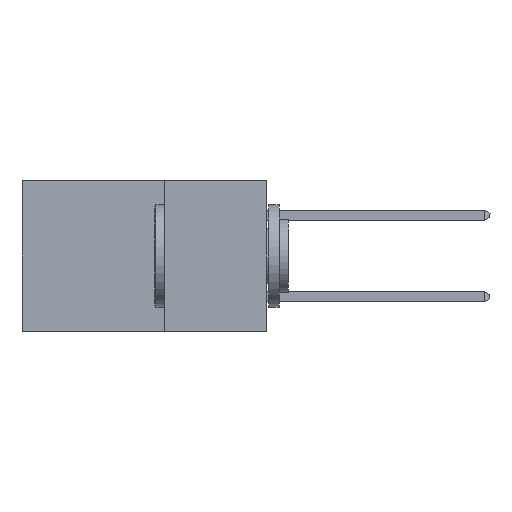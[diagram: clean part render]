
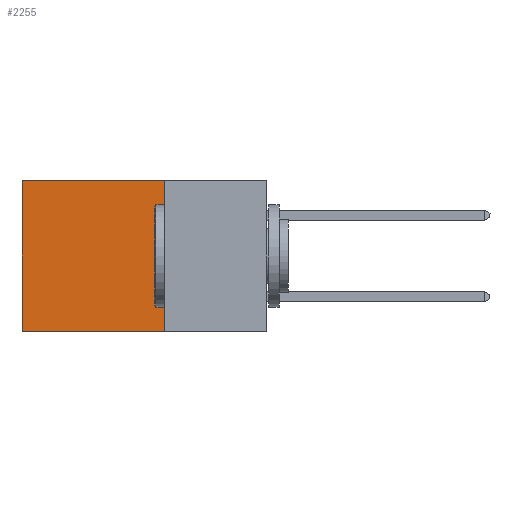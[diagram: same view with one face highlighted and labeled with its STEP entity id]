
A CAD part, left-side view. The second image highlights one B-rep face of the part: STEP entity #2255.
In plain terms, the highlighted planar face has unit normal (-1, 0, 0).
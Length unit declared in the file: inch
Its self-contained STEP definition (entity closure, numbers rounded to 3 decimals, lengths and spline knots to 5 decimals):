
#316 = ORIENTED_EDGE ( 'NONE', *, *, #842, .T. ) ;
#406 = ORIENTED_EDGE ( 'NONE', *, *, #447, .F. ) ;
#423 = VECTOR ( 'NONE', #3662, 39.37008 ) ;
#447 = EDGE_CURVE ( 'NONE', #13994, #11689, #9761, .T. ) ;
#842 = EDGE_CURVE ( 'NONE', #3643, #11689, #13618, .T. ) ;
#846 = VECTOR ( 'NONE', #10991, 39.37008 ) ;
#1042 = LINE ( 'NONE', #2290, #7118 ) ;
#1079 = CARTESIAN_POINT ( 'NONE',  ( 0.2875, 0.6, -0.37 ) ) ;
#1954 = VERTEX_POINT ( 'NONE', #15125 ) ;
#2255 = ADVANCED_FACE ( 'NONE', ( #5760 ), #12206, .F. ) ;
#2290 = CARTESIAN_POINT ( 'NONE',  ( 0.2875, 0.25, 0. ) ) ;
#2698 = AXIS2_PLACEMENT_3D ( 'NONE', #12236, #12100, #12096 ) ;
#3304 = ORIENTED_EDGE ( 'NONE', *, *, #9925, .T. ) ;
#3643 = VERTEX_POINT ( 'NONE', #15155 ) ;
#3662 = DIRECTION ( 'NONE',  ( 0., 1., 0. ) ) ;
#3919 = CARTESIAN_POINT ( 'NONE',  ( 0.2875, 0.25, -0.37 ) ) ;
#4709 = CARTESIAN_POINT ( 'NONE',  ( 0.2875, 0.25, -0.37 ) ) ;
#5433 = CARTESIAN_POINT ( 'NONE',  ( 0.2875, 0.25, 0. ) ) ;
#5760 = FACE_OUTER_BOUND ( 'NONE', #8835, .T. ) ;
#7118 = VECTOR ( 'NONE', #11857, 39.37008 ) ;
#8039 = LINE ( 'NONE', #5433, #11234 ) ;
#8835 = EDGE_LOOP ( 'NONE', ( #316, #406, #9930, #3304 ) ) ;
#9761 = LINE ( 'NONE', #3919, #423 ) ;
#9925 = EDGE_CURVE ( 'NONE', #1954, #3643, #1042, .T. ) ;
#9930 = ORIENTED_EDGE ( 'NONE', *, *, #14927, .F. ) ;
#10421 = CARTESIAN_POINT ( 'NONE',  ( 0.2875, 0.6, 0. ) ) ;
#10991 = DIRECTION ( 'NONE',  ( 0., 0., -1. ) ) ;
#11234 = VECTOR ( 'NONE', #13755, 39.37008 ) ;
#11689 = VERTEX_POINT ( 'NONE', #1079 ) ;
#11857 = DIRECTION ( 'NONE',  ( 0., 1., 0. ) ) ;
#12096 = DIRECTION ( 'NONE',  ( 0., 0., -1. ) ) ;
#12100 = DIRECTION ( 'NONE',  ( 1., 0., 0. ) ) ;
#12206 = PLANE ( 'NONE',  #2698 ) ;
#12236 = CARTESIAN_POINT ( 'NONE',  ( 0.2875, 0.25, 0. ) ) ;
#13618 = LINE ( 'NONE', #10421, #846 ) ;
#13755 = DIRECTION ( 'NONE',  ( 0., 0., -1. ) ) ;
#13994 = VERTEX_POINT ( 'NONE', #4709 ) ;
#14927 = EDGE_CURVE ( 'NONE', #1954, #13994, #8039, .T. ) ;
#15125 = CARTESIAN_POINT ( 'NONE',  ( 0.2875, 0.25, 0. ) ) ;
#15155 = CARTESIAN_POINT ( 'NONE',  ( 0.2875, 0.6, 0. ) ) ;
